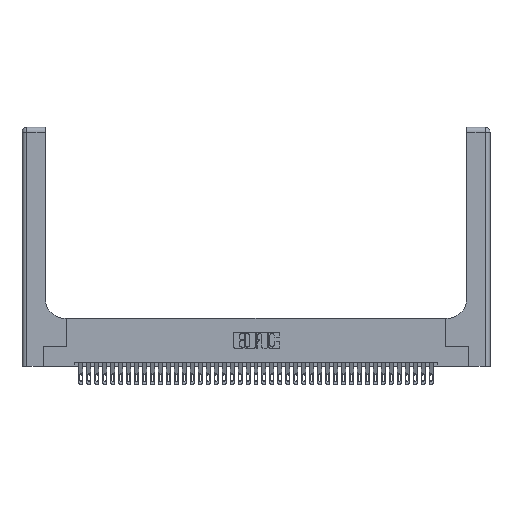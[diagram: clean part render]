
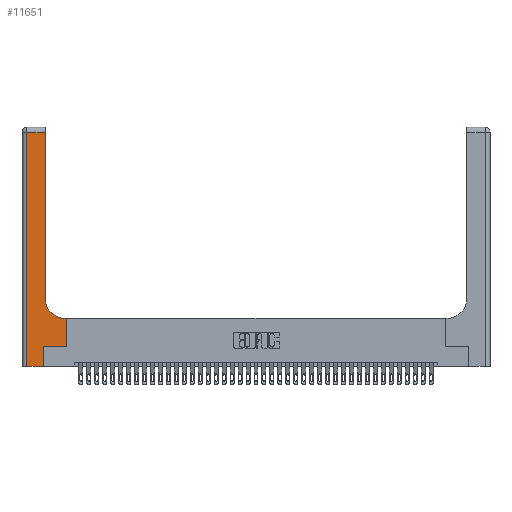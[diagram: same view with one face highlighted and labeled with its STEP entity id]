
A CAD part, top view. The second image highlights one B-rep face of the part: STEP entity #11651.
In plain terms, the highlighted planar face has unit normal (0, 0, 1).
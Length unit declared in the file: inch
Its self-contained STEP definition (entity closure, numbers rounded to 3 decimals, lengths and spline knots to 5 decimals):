
#342 = AXIS2_PLACEMENT_3D ( 'NONE', #37276, #6200, #28018 ) ;
#357 = EDGE_CURVE ( 'NONE', #4207, #18440, #29873, .T. ) ;
#936 = ORIENTED_EDGE ( 'NONE', *, *, #27306, .T. ) ;
#1380 = ORIENTED_EDGE ( 'NONE', *, *, #8764, .T. ) ;
#1655 = CARTESIAN_POINT ( 'NONE',  ( 0.269, 0., 0.37 ) ) ;
#3043 = PLANE ( 'NONE',  #342 ) ;
#3371 = ORIENTED_EDGE ( 'NONE', *, *, #39415, .T. ) ;
#3806 = CARTESIAN_POINT ( 'NONE',  ( 0.269, 0.25, 0.37 ) ) ;
#3857 = VERTEX_POINT ( 'NONE', #20167 ) ;
#4207 = VERTEX_POINT ( 'NONE', #6055 ) ;
#4812 = DIRECTION ( 'NONE',  ( 0., 1., 0. ) ) ;
#5495 = CARTESIAN_POINT ( 'NONE',  ( 0.269, 0., 0.37 ) ) ;
#5926 = LINE ( 'NONE', #14637, #21550 ) ;
#5936 = VERTEX_POINT ( 'NONE', #25643 ) ;
#6055 = CARTESIAN_POINT ( 'NONE',  ( 0.5585, 0.6, 0.37 ) ) ;
#6091 = DIRECTION ( 'NONE',  ( 0., 0., -1. ) ) ;
#6200 = DIRECTION ( 'NONE',  ( 0., 0., -1. ) ) ;
#6722 = LINE ( 'NONE', #12924, #17016 ) ;
#7251 = EDGE_CURVE ( 'NONE', #20786, #5936, #40169, .T. ) ;
#8501 = LINE ( 'NONE', #8615, #15825 ) ;
#8615 = CARTESIAN_POINT ( 'NONE',  ( 0.5585, 0.25, 0.37 ) ) ;
#8764 = EDGE_CURVE ( 'NONE', #36640, #14713, #5926, .T. ) ;
#10165 = LINE ( 'NONE', #27632, #17532 ) ;
#11330 = CARTESIAN_POINT ( 'NONE',  ( 0.2915, 0.6, 0.37 ) ) ;
#11651 = ADVANCED_FACE ( 'NONE', ( #20151 ), #3043, .F. ) ;
#12121 = DIRECTION ( 'NONE',  ( 1., 0., 0. ) ) ;
#12408 = VERTEX_POINT ( 'NONE', #22656 ) ;
#12697 = ORIENTED_EDGE ( 'NONE', *, *, #30135, .T. ) ;
#12924 = CARTESIAN_POINT ( 'NONE',  ( 0., 2.94, 0.37 ) ) ;
#13288 = VECTOR ( 'NONE', #23699, 39.37008 ) ;
#13741 = EDGE_LOOP ( 'NONE', ( #15678, #936, #1380, #3371, #20022, #12697, #38516, #14644, #32170 ) ) ;
#14637 = CARTESIAN_POINT ( 'NONE',  ( 0.06, 3., 0.37 ) ) ;
#14644 = ORIENTED_EDGE ( 'NONE', *, *, #357, .T. ) ;
#14713 = VERTEX_POINT ( 'NONE', #15875 ) ;
#15302 = VECTOR ( 'NONE', #35049, 39.37008 ) ;
#15345 = VECTOR ( 'NONE', #22731, 39.37008 ) ;
#15678 = ORIENTED_EDGE ( 'NONE', *, *, #7251, .T. ) ;
#15825 = VECTOR ( 'NONE', #36659, 39.37008 ) ;
#15875 = CARTESIAN_POINT ( 'NONE',  ( 0.06, 0., 0.37 ) ) ;
#16289 = EDGE_CURVE ( 'NONE', #18440, #20786, #16875, .T. ) ;
#16344 = CARTESIAN_POINT ( 'NONE',  ( 0.5415, 0.6, 0.37 ) ) ;
#16875 = CIRCLE ( 'NONE', #20049, 0.25 ) ;
#17016 = VECTOR ( 'NONE', #34729, 39.37008 ) ;
#17532 = VECTOR ( 'NONE', #12121, 39.37008 ) ;
#18440 = VERTEX_POINT ( 'NONE', #16344 ) ;
#19641 = CARTESIAN_POINT ( 'NONE',  ( 0.06, 2.94, 0.37 ) ) ;
#20022 = ORIENTED_EDGE ( 'NONE', *, *, #29753, .T. ) ;
#20049 = AXIS2_PLACEMENT_3D ( 'NONE', #24747, #6091, #27909 ) ;
#20151 = FACE_OUTER_BOUND ( 'NONE', #13741, .T. ) ;
#20167 = CARTESIAN_POINT ( 'NONE',  ( 0.269, 0.25, 0.37 ) ) ;
#20237 = VECTOR ( 'NONE', #4812, 39.37008 ) ;
#20786 = VERTEX_POINT ( 'NONE', #25413 ) ;
#21180 = LINE ( 'NONE', #1655, #20237 ) ;
#21550 = VECTOR ( 'NONE', #39563, 39.37008 ) ;
#22656 = CARTESIAN_POINT ( 'NONE',  ( 0.5585, 0.25, 0.37 ) ) ;
#22731 = DIRECTION ( 'NONE',  ( 0., 1., 0. ) ) ;
#23570 = LINE ( 'NONE', #3806, #15302 ) ;
#23699 = DIRECTION ( 'NONE',  ( -1., 0., 0. ) ) ;
#24747 = CARTESIAN_POINT ( 'NONE',  ( 0.5415, 0.85, 0.37 ) ) ;
#25413 = CARTESIAN_POINT ( 'NONE',  ( 0.2915, 0.85, 0.37 ) ) ;
#25643 = CARTESIAN_POINT ( 'NONE',  ( 0.2915, 2.94, 0.37 ) ) ;
#25836 = CARTESIAN_POINT ( 'NONE',  ( 0.2915, 3., 0.37 ) ) ;
#27306 = EDGE_CURVE ( 'NONE', #5936, #36640, #6722, .T. ) ;
#27632 = CARTESIAN_POINT ( 'NONE',  ( 0., 0., 0.37 ) ) ;
#27909 = DIRECTION ( 'NONE',  ( 1., 0., 0. ) ) ;
#28018 = DIRECTION ( 'NONE',  ( -1., 0., 0. ) ) ;
#29753 = EDGE_CURVE ( 'NONE', #40134, #3857, #21180, .T. ) ;
#29873 = LINE ( 'NONE', #11330, #13288 ) ;
#30135 = EDGE_CURVE ( 'NONE', #3857, #12408, #23570, .T. ) ;
#32170 = ORIENTED_EDGE ( 'NONE', *, *, #16289, .T. ) ;
#34729 = DIRECTION ( 'NONE',  ( -1., 0., 0. ) ) ;
#35049 = DIRECTION ( 'NONE',  ( 1., 0., 0. ) ) ;
#36266 = EDGE_CURVE ( 'NONE', #12408, #4207, #8501, .T. ) ;
#36640 = VERTEX_POINT ( 'NONE', #19641 ) ;
#36659 = DIRECTION ( 'NONE',  ( 0., 1., 0. ) ) ;
#37276 = CARTESIAN_POINT ( 'NONE',  ( 0., 3., 0.37 ) ) ;
#38516 = ORIENTED_EDGE ( 'NONE', *, *, #36266, .T. ) ;
#39415 = EDGE_CURVE ( 'NONE', #14713, #40134, #10165, .T. ) ;
#39563 = DIRECTION ( 'NONE',  ( 0., -1., 0. ) ) ;
#40134 = VERTEX_POINT ( 'NONE', #5495 ) ;
#40169 = LINE ( 'NONE', #25836, #15345 ) ;
